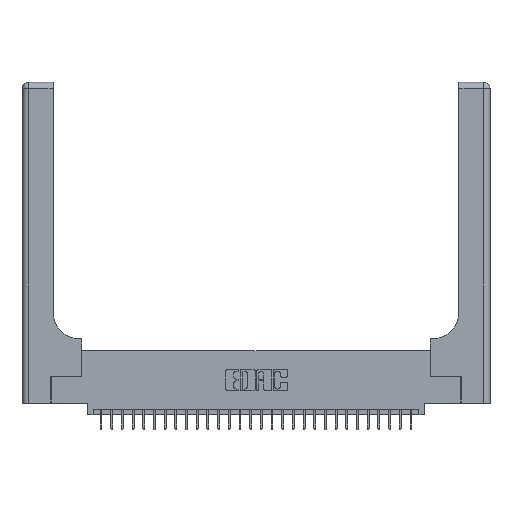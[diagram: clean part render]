
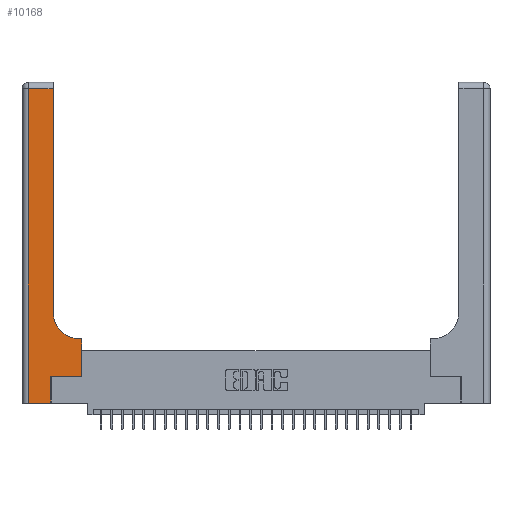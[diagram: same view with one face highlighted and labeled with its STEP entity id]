
A CAD part, top view. The second image highlights one B-rep face of the part: STEP entity #10168.
In plain terms, the highlighted planar face has unit normal (0, 0, 1).
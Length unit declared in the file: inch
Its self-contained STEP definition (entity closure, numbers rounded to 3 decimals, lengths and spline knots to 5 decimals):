
#105 = ORIENTED_EDGE ( 'NONE', *, *, #22796, .T. ) ;
#323 = LINE ( 'NONE', #28508, #13748 ) ;
#373 = CARTESIAN_POINT ( 'NONE',  ( 0.5585, 0.6, 0.37 ) ) ;
#499 = VERTEX_POINT ( 'NONE', #20922 ) ;
#1114 = CARTESIAN_POINT ( 'NONE',  ( 0.269, 0.25, 0.37 ) ) ;
#1558 = DIRECTION ( 'NONE',  ( -1., 0., 0. ) ) ;
#2976 = LINE ( 'NONE', #1114, #19999 ) ;
#3296 = VECTOR ( 'NONE', #1558, 39.37008 ) ;
#3502 = CARTESIAN_POINT ( 'NONE',  ( 0.06, 2.94, 0.37 ) ) ;
#4636 = CIRCLE ( 'NONE', #16899, 0.25 ) ;
#4668 = ORIENTED_EDGE ( 'NONE', *, *, #11915, .T. ) ;
#5177 = LINE ( 'NONE', #21678, #11961 ) ;
#5419 = EDGE_CURVE ( 'NONE', #499, #13736, #18100, .T. ) ;
#5530 = CARTESIAN_POINT ( 'NONE',  ( 0.2915, 2.94, 0.37 ) ) ;
#5680 = DIRECTION ( 'NONE',  ( -1., 0., 0. ) ) ;
#6258 = VECTOR ( 'NONE', #28971, 39.37008 ) ;
#6345 = DIRECTION ( 'NONE',  ( 1., 0., 0. ) ) ;
#6434 = ORIENTED_EDGE ( 'NONE', *, *, #22683, .T. ) ;
#6696 = DIRECTION ( 'NONE',  ( 0., 1., 0. ) ) ;
#6900 = EDGE_CURVE ( 'NONE', #13736, #17259, #323, .T. ) ;
#7276 = LINE ( 'NONE', #28801, #24429 ) ;
#8301 = VECTOR ( 'NONE', #22480, 39.37008 ) ;
#9471 = CARTESIAN_POINT ( 'NONE',  ( 0.269, 0.25, 0.37 ) ) ;
#9487 = EDGE_CURVE ( 'NONE', #26554, #16231, #16061, .T. ) ;
#9829 = ORIENTED_EDGE ( 'NONE', *, *, #20478, .T. ) ;
#10168 = ADVANCED_FACE ( 'NONE', ( #24839 ), #24685, .F. ) ;
#11915 = EDGE_CURVE ( 'NONE', #27345, #499, #5177, .T. ) ;
#11961 = VECTOR ( 'NONE', #18848, 39.37008 ) ;
#12088 = VERTEX_POINT ( 'NONE', #27887 ) ;
#12731 = VERTEX_POINT ( 'NONE', #16393 ) ;
#13736 = VERTEX_POINT ( 'NONE', #20596 ) ;
#13748 = VECTOR ( 'NONE', #21009, 39.37008 ) ;
#14363 = CARTESIAN_POINT ( 'NONE',  ( 0.5585, 0.25, 0.37 ) ) ;
#14861 = VECTOR ( 'NONE', #6696, 39.37008 ) ;
#15453 = ORIENTED_EDGE ( 'NONE', *, *, #19234, .T. ) ;
#15527 = VERTEX_POINT ( 'NONE', #373 ) ;
#16061 = LINE ( 'NONE', #23076, #14861 ) ;
#16177 = DIRECTION ( 'NONE',  ( -1., 0., 0. ) ) ;
#16231 = VERTEX_POINT ( 'NONE', #5530 ) ;
#16393 = CARTESIAN_POINT ( 'NONE',  ( 0.5585, 0.25, 0.37 ) ) ;
#16899 = AXIS2_PLACEMENT_3D ( 'NONE', #28379, #27901, #25726 ) ;
#16978 = ORIENTED_EDGE ( 'NONE', *, *, #5419, .T. ) ;
#17254 = EDGE_CURVE ( 'NONE', #12088, #26554, #4636, .T. ) ;
#17259 = VERTEX_POINT ( 'NONE', #9471 ) ;
#17405 = EDGE_LOOP ( 'NONE', ( #19864, #15453, #4668, #16978, #29620, #105, #6434, #9829, #26407 ) ) ;
#18100 = LINE ( 'NONE', #20437, #8301 ) ;
#18733 = AXIS2_PLACEMENT_3D ( 'NONE', #20136, #29669, #5680 ) ;
#18848 = DIRECTION ( 'NONE',  ( 0., -1., 0. ) ) ;
#19234 = EDGE_CURVE ( 'NONE', #16231, #27345, #7276, .T. ) ;
#19864 = ORIENTED_EDGE ( 'NONE', *, *, #9487, .T. ) ;
#19999 = VECTOR ( 'NONE', #6345, 39.37008 ) ;
#20136 = CARTESIAN_POINT ( 'NONE',  ( 0., 3., 0.37 ) ) ;
#20437 = CARTESIAN_POINT ( 'NONE',  ( 0., 0., 0.37 ) ) ;
#20478 = EDGE_CURVE ( 'NONE', #15527, #12088, #22868, .T. ) ;
#20596 = CARTESIAN_POINT ( 'NONE',  ( 0.269, 0., 0.37 ) ) ;
#20922 = CARTESIAN_POINT ( 'NONE',  ( 0.06, 0., 0.37 ) ) ;
#21009 = DIRECTION ( 'NONE',  ( 0., 1., 0. ) ) ;
#21113 = CARTESIAN_POINT ( 'NONE',  ( 0.2915, 0.85, 0.37 ) ) ;
#21678 = CARTESIAN_POINT ( 'NONE',  ( 0.06, 3., 0.37 ) ) ;
#22480 = DIRECTION ( 'NONE',  ( 1., 0., 0. ) ) ;
#22683 = EDGE_CURVE ( 'NONE', #12731, #15527, #28679, .T. ) ;
#22796 = EDGE_CURVE ( 'NONE', #17259, #12731, #2976, .T. ) ;
#22868 = LINE ( 'NONE', #27553, #3296 ) ;
#23076 = CARTESIAN_POINT ( 'NONE',  ( 0.2915, 3., 0.37 ) ) ;
#24429 = VECTOR ( 'NONE', #16177, 39.37008 ) ;
#24685 = PLANE ( 'NONE',  #18733 ) ;
#24839 = FACE_OUTER_BOUND ( 'NONE', #17405, .T. ) ;
#25726 = DIRECTION ( 'NONE',  ( 1., 0., 0. ) ) ;
#26407 = ORIENTED_EDGE ( 'NONE', *, *, #17254, .T. ) ;
#26554 = VERTEX_POINT ( 'NONE', #21113 ) ;
#27345 = VERTEX_POINT ( 'NONE', #3502 ) ;
#27553 = CARTESIAN_POINT ( 'NONE',  ( 0.2915, 0.6, 0.37 ) ) ;
#27887 = CARTESIAN_POINT ( 'NONE',  ( 0.5415, 0.6, 0.37 ) ) ;
#27901 = DIRECTION ( 'NONE',  ( 0., 0., -1. ) ) ;
#28379 = CARTESIAN_POINT ( 'NONE',  ( 0.5415, 0.85, 0.37 ) ) ;
#28508 = CARTESIAN_POINT ( 'NONE',  ( 0.269, 0., 0.37 ) ) ;
#28679 = LINE ( 'NONE', #14363, #6258 ) ;
#28801 = CARTESIAN_POINT ( 'NONE',  ( 0., 2.94, 0.37 ) ) ;
#28971 = DIRECTION ( 'NONE',  ( 0., 1., 0. ) ) ;
#29620 = ORIENTED_EDGE ( 'NONE', *, *, #6900, .T. ) ;
#29669 = DIRECTION ( 'NONE',  ( 0., 0., -1. ) ) ;
